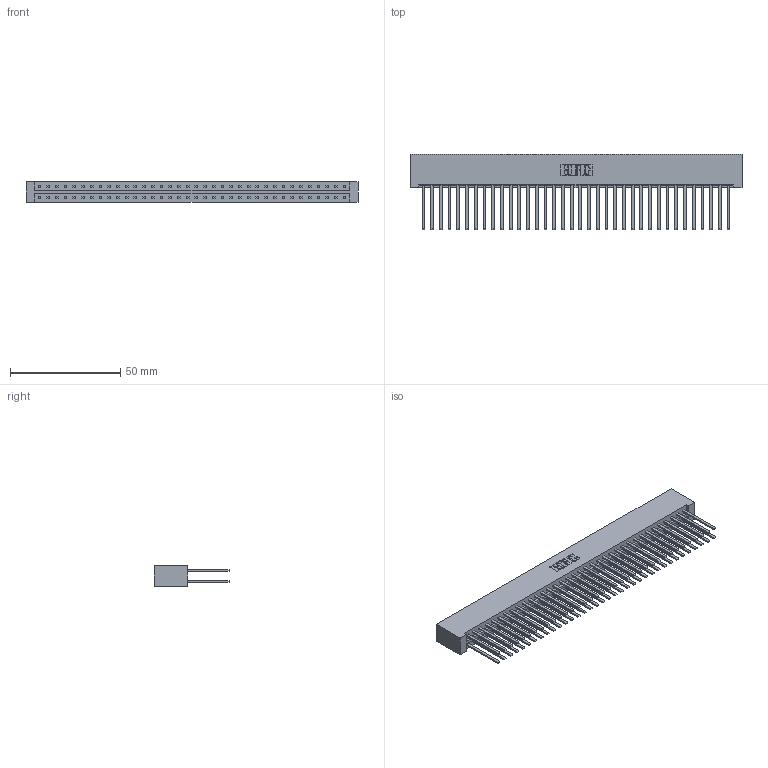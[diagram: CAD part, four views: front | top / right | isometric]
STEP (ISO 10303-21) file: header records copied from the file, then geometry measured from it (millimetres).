
FILE_DESCRIPTION (( 'STEP AP203' ), '1' );
FILE_NAME ('333-072-544-201.STEP', '2018-08-04T20:57:29', ( '' ), ( '' ), 'SwSTEP 2.0', 'SolidWorks 2016', '' );
FILE_SCHEMA (( 'CONFIG_CONTROL_DESIGN' ));
Length unit declared in the file: inch
Products named in the file (3): 333-072-544-201; 333 Part_Lugless; 345-292-001_345-293-144
Assembly tree (73 placements, depth 2):
  333-072-544-201
    333 Part_Lugless
    345-292-001_345-293-144  x72
Bounding box: 150.9 x 34.3 x 9.4 mm (x, y, z)
Volume: 16991.6 mm3; surface area: 23297.9 mm2
Topology: 73 solids, 73 shells, 3418 faces, 10151 edges, 6670 vertices
Faces by surface type: plane 2370, cylinder 1048
Entity records: 23475 total; most frequent: CARTESIAN_POINT 3894, ORIENTED_EDGE 3830, DIRECTION 3327, EDGE_CURVE 1915, VECTOR 1799, LINE 1799, VERTEX_POINT 1274, AXIS2_PLACEMENT_3D 764
